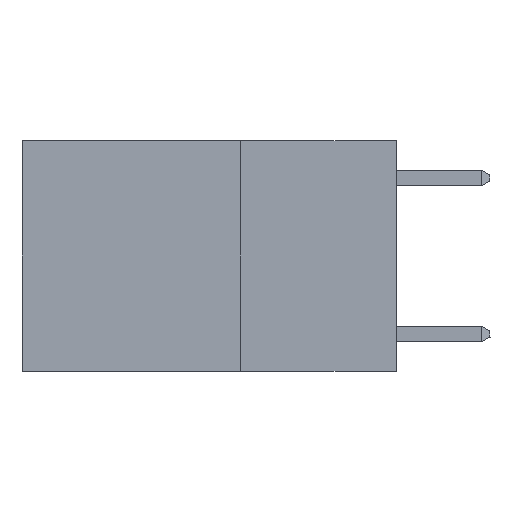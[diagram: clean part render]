
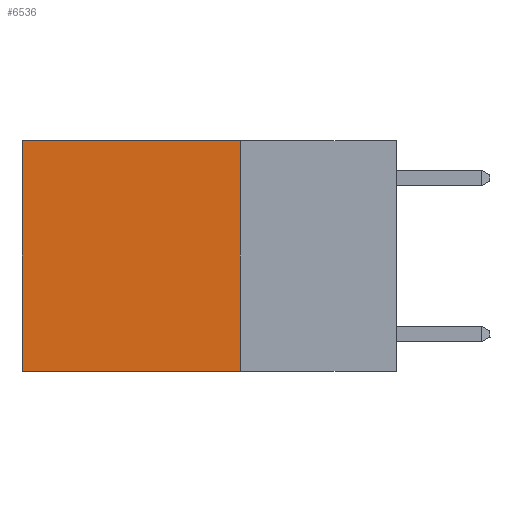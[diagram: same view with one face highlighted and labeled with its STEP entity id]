
A CAD part, left-side view. The second image highlights one B-rep face of the part: STEP entity #6536.
In plain terms, the highlighted planar face has unit normal (-1, 0, 0).
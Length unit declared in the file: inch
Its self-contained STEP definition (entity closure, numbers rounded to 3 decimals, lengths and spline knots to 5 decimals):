
#72 = EDGE_CURVE ( 'NONE', #9856, #10031, #9183, .T. ) ;
#90 = EDGE_CURVE ( 'NONE', #10031, #8420, #5867, .T. ) ;
#239 = VECTOR ( 'NONE', #10162, 39.37008 ) ;
#1058 = CARTESIAN_POINT ( 'NONE',  ( 0.2625, 0.25, 0. ) ) ;
#1144 = CARTESIAN_POINT ( 'NONE',  ( 0.2625, 0.6, 0. ) ) ;
#1604 = LINE ( 'NONE', #10097, #239 ) ;
#1743 = CARTESIAN_POINT ( 'NONE',  ( 0.2625, 0.25, 0. ) ) ;
#2221 = DIRECTION ( 'NONE',  ( 0., 1., 0. ) ) ;
#2334 = ORIENTED_EDGE ( 'NONE', *, *, #90, .F. ) ;
#2453 = VECTOR ( 'NONE', #2221, 39.37008 ) ;
#4660 = ORIENTED_EDGE ( 'NONE', *, *, #4869, .T. ) ;
#4764 = CARTESIAN_POINT ( 'NONE',  ( 0.2625, 0.6, -0.37 ) ) ;
#4869 = EDGE_CURVE ( 'NONE', #7371, #8420, #1604, .T. ) ;
#5135 = EDGE_CURVE ( 'NONE', #9856, #7371, #11920, .T. ) ;
#5368 = DIRECTION ( 'NONE',  ( 0., 0., -1. ) ) ;
#5867 = LINE ( 'NONE', #8249, #10876 ) ;
#6043 = CARTESIAN_POINT ( 'NONE',  ( 0.2625, 0.25, 0. ) ) ;
#6074 = DIRECTION ( 'NONE',  ( 0., 0., -1. ) ) ;
#6158 = FACE_OUTER_BOUND ( 'NONE', #6923, .T. ) ;
#6361 = PLANE ( 'NONE',  #7241 ) ;
#6536 = ADVANCED_FACE ( 'NONE', ( #6158 ), #6361, .F. ) ;
#6923 = EDGE_LOOP ( 'NONE', ( #4660, #2334, #11688, #13410 ) ) ;
#7241 = AXIS2_PLACEMENT_3D ( 'NONE', #1058, #8552, #5368 ) ;
#7371 = VERTEX_POINT ( 'NONE', #1144 ) ;
#8249 = CARTESIAN_POINT ( 'NONE',  ( 0.2625, 0.25, -0.37 ) ) ;
#8420 = VERTEX_POINT ( 'NONE', #4764 ) ;
#8552 = DIRECTION ( 'NONE',  ( 1., 0., 0. ) ) ;
#8608 = CARTESIAN_POINT ( 'NONE',  ( 0.2625, 0.25, 0. ) ) ;
#9183 = LINE ( 'NONE', #1743, #13387 ) ;
#9856 = VERTEX_POINT ( 'NONE', #6043 ) ;
#9862 = CARTESIAN_POINT ( 'NONE',  ( 0.2625, 0.25, -0.37 ) ) ;
#10031 = VERTEX_POINT ( 'NONE', #9862 ) ;
#10097 = CARTESIAN_POINT ( 'NONE',  ( 0.2625, 0.6, 0. ) ) ;
#10106 = DIRECTION ( 'NONE',  ( 0., 1., 0. ) ) ;
#10162 = DIRECTION ( 'NONE',  ( 0., 0., -1. ) ) ;
#10876 = VECTOR ( 'NONE', #10106, 39.37008 ) ;
#11688 = ORIENTED_EDGE ( 'NONE', *, *, #72, .F. ) ;
#11920 = LINE ( 'NONE', #8608, #2453 ) ;
#13387 = VECTOR ( 'NONE', #6074, 39.37008 ) ;
#13410 = ORIENTED_EDGE ( 'NONE', *, *, #5135, .T. ) ;
